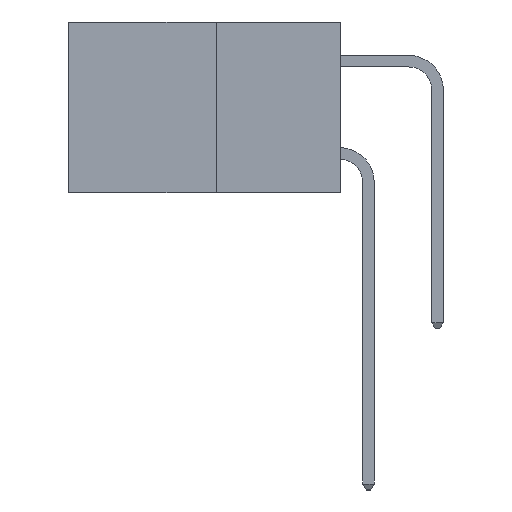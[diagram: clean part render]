
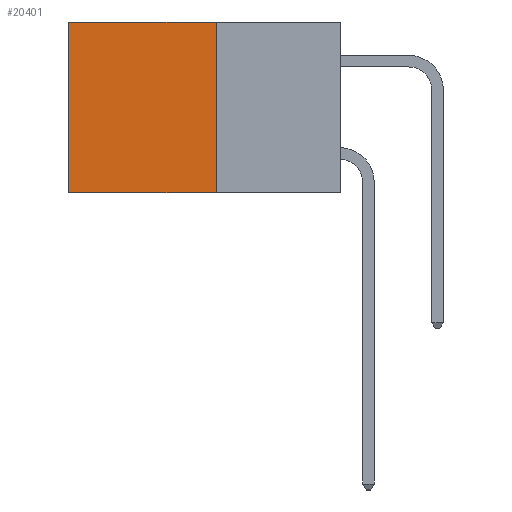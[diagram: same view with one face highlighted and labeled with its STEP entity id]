
A CAD part, left-side view. The second image highlights one B-rep face of the part: STEP entity #20401.
In plain terms, the highlighted planar face has unit normal (-1, 0, 0).
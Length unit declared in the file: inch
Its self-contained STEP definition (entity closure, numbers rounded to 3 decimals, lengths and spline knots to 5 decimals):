
#96 = CARTESIAN_POINT ( 'NONE',  ( 0.277, 0.27, -0.37 ) ) ;
#194 = PLANE ( 'NONE',  #19884 ) ;
#481 = VERTEX_POINT ( 'NONE', #18095 ) ;
#1395 = VECTOR ( 'NONE', #16246, 39.37008 ) ;
#2084 = CARTESIAN_POINT ( 'NONE',  ( 0.277, 0.27, -0.37 ) ) ;
#2192 = VECTOR ( 'NONE', #19747, 39.37008 ) ;
#3801 = DIRECTION ( 'NONE',  ( 1., 0., 0. ) ) ;
#4098 = LINE ( 'NONE', #96, #7405 ) ;
#4099 = CARTESIAN_POINT ( 'NONE',  ( 0.277, 0.59, -0.37 ) ) ;
#4107 = EDGE_CURVE ( 'NONE', #16553, #7586, #14436, .T. ) ;
#6340 = EDGE_CURVE ( 'NONE', #18245, #481, #4098, .T. ) ;
#6727 = ORIENTED_EDGE ( 'NONE', *, *, #4107, .T. ) ;
#7405 = VECTOR ( 'NONE', #8438, 39.37008 ) ;
#7586 = VERTEX_POINT ( 'NONE', #20538 ) ;
#8064 = FACE_OUTER_BOUND ( 'NONE', #14655, .T. ) ;
#8438 = DIRECTION ( 'NONE',  ( 0., 1., 0. ) ) ;
#9176 = VECTOR ( 'NONE', #10993, 39.37008 ) ;
#9720 = EDGE_CURVE ( 'NONE', #16553, #18245, #14011, .T. ) ;
#10285 = LINE ( 'NONE', #4099, #2192 ) ;
#10550 = ORIENTED_EDGE ( 'NONE', *, *, #19851, .T. ) ;
#10993 = DIRECTION ( 'NONE',  ( 0., 0., -1. ) ) ;
#11612 = ORIENTED_EDGE ( 'NONE', *, *, #6340, .F. ) ;
#13960 = ORIENTED_EDGE ( 'NONE', *, *, #9720, .F. ) ;
#14011 = LINE ( 'NONE', #18845, #9176 ) ;
#14436 = LINE ( 'NONE', #16297, #1395 ) ;
#14655 = EDGE_LOOP ( 'NONE', ( #10550, #11612, #13960, #6727 ) ) ;
#14747 = CARTESIAN_POINT ( 'NONE',  ( 0.277, 0.27, -0.37 ) ) ;
#15109 = DIRECTION ( 'NONE',  ( 0., 0., -1. ) ) ;
#16246 = DIRECTION ( 'NONE',  ( 0., 1., 0. ) ) ;
#16297 = CARTESIAN_POINT ( 'NONE',  ( 0.277, 0.27, 0. ) ) ;
#16434 = CARTESIAN_POINT ( 'NONE',  ( 0.277, 0.27, 0. ) ) ;
#16553 = VERTEX_POINT ( 'NONE', #16434 ) ;
#18095 = CARTESIAN_POINT ( 'NONE',  ( 0.277, 0.59, -0.37 ) ) ;
#18245 = VERTEX_POINT ( 'NONE', #14747 ) ;
#18845 = CARTESIAN_POINT ( 'NONE',  ( 0.277, 0.27, -0.37 ) ) ;
#19747 = DIRECTION ( 'NONE',  ( 0., 0., -1. ) ) ;
#19851 = EDGE_CURVE ( 'NONE', #7586, #481, #10285, .T. ) ;
#19884 = AXIS2_PLACEMENT_3D ( 'NONE', #2084, #3801, #15109 ) ;
#20401 = ADVANCED_FACE ( 'NONE', ( #8064 ), #194, .F. ) ;
#20538 = CARTESIAN_POINT ( 'NONE',  ( 0.277, 0.59, 0. ) ) ;
